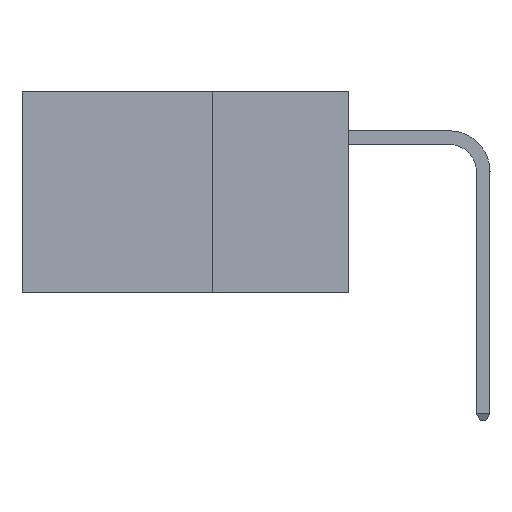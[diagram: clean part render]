
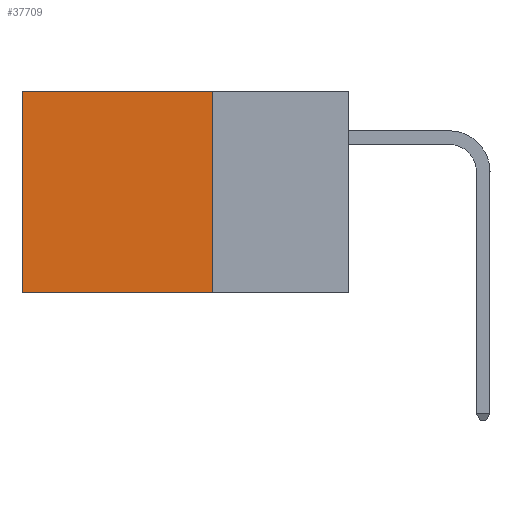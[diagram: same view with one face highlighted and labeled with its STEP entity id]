
A CAD part, left-side view. The second image highlights one B-rep face of the part: STEP entity #37709.
In plain terms, the highlighted planar face has unit normal (-1, 0, 0).
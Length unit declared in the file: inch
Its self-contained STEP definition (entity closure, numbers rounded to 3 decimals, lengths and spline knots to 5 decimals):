
#316 = CARTESIAN_POINT ( 'NONE',  ( 0.2875, 0.25, 0. ) ) ;
#540 = EDGE_CURVE ( 'NONE', #2411, #13515, #8812, .T. ) ;
#976 = AXIS2_PLACEMENT_3D ( 'NONE', #26393, #39225, #23534 ) ;
#989 = PLANE ( 'NONE',  #976 ) ;
#1694 = VERTEX_POINT ( 'NONE', #10416 ) ;
#2411 = VERTEX_POINT ( 'NONE', #34519 ) ;
#5952 = VERTEX_POINT ( 'NONE', #16929 ) ;
#6998 = CARTESIAN_POINT ( 'NONE',  ( 0.2875, 0.6, -0.37 ) ) ;
#8116 = EDGE_CURVE ( 'NONE', #5952, #13515, #40110, .T. ) ;
#8738 = CARTESIAN_POINT ( 'NONE',  ( 0.2875, 0.25, 0. ) ) ;
#8812 = LINE ( 'NONE', #16271, #11216 ) ;
#10416 = CARTESIAN_POINT ( 'NONE',  ( 0.2875, 0.25, 0. ) ) ;
#11216 = VECTOR ( 'NONE', #34639, 39.37008 ) ;
#11769 = FACE_OUTER_BOUND ( 'NONE', #17110, .T. ) ;
#13314 = DIRECTION ( 'NONE',  ( 0., 0., -1. ) ) ;
#13456 = ORIENTED_EDGE ( 'NONE', *, *, #24730, .F. ) ;
#13515 = VERTEX_POINT ( 'NONE', #6998 ) ;
#15343 = EDGE_CURVE ( 'NONE', #1694, #5952, #30436, .T. ) ;
#16271 = CARTESIAN_POINT ( 'NONE',  ( 0.2875, 0.25, -0.37 ) ) ;
#16929 = CARTESIAN_POINT ( 'NONE',  ( 0.2875, 0.6, 0. ) ) ;
#17110 = EDGE_LOOP ( 'NONE', ( #29578, #25672, #13456, #18355 ) ) ;
#18355 = ORIENTED_EDGE ( 'NONE', *, *, #15343, .T. ) ;
#21032 = LINE ( 'NONE', #316, #28819 ) ;
#22573 = CARTESIAN_POINT ( 'NONE',  ( 0.2875, 0.6, 0. ) ) ;
#23109 = VECTOR ( 'NONE', #24688, 39.37008 ) ;
#23534 = DIRECTION ( 'NONE',  ( 0., 0., -1. ) ) ;
#24688 = DIRECTION ( 'NONE',  ( 0., 1., 0. ) ) ;
#24730 = EDGE_CURVE ( 'NONE', #1694, #2411, #21032, .T. ) ;
#25672 = ORIENTED_EDGE ( 'NONE', *, *, #540, .F. ) ;
#26393 = CARTESIAN_POINT ( 'NONE',  ( 0.2875, 0.25, 0. ) ) ;
#28819 = VECTOR ( 'NONE', #28843, 39.37008 ) ;
#28843 = DIRECTION ( 'NONE',  ( 0., 0., -1. ) ) ;
#29578 = ORIENTED_EDGE ( 'NONE', *, *, #8116, .T. ) ;
#30436 = LINE ( 'NONE', #8738, #23109 ) ;
#34519 = CARTESIAN_POINT ( 'NONE',  ( 0.2875, 0.25, -0.37 ) ) ;
#34639 = DIRECTION ( 'NONE',  ( 0., 1., 0. ) ) ;
#35710 = VECTOR ( 'NONE', #13314, 39.37008 ) ;
#37709 = ADVANCED_FACE ( 'NONE', ( #11769 ), #989, .F. ) ;
#39225 = DIRECTION ( 'NONE',  ( 1., 0., 0. ) ) ;
#40110 = LINE ( 'NONE', #22573, #35710 ) ;
